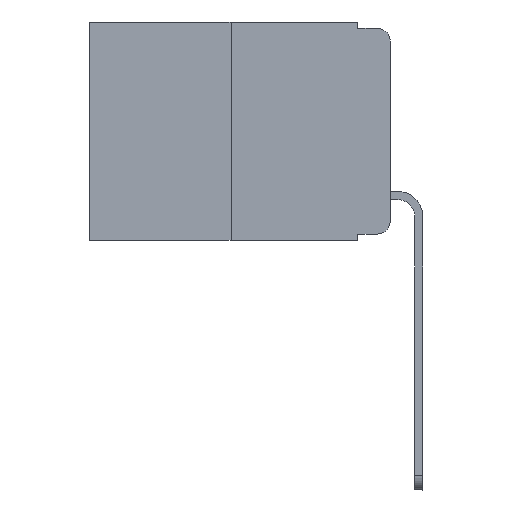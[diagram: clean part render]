
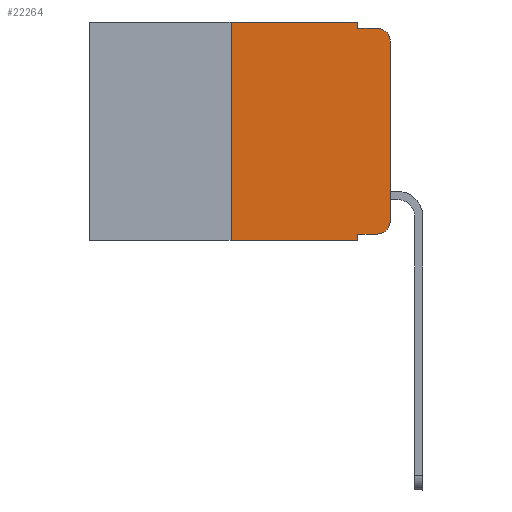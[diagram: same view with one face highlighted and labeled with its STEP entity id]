
A CAD part, left-side view. The second image highlights one B-rep face of the part: STEP entity #22264.
In plain terms, the highlighted planar face has unit normal (-1, 0, 0).
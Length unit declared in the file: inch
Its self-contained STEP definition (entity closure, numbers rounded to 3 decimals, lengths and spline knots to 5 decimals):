
#42 = EDGE_CURVE ( 'NONE', #20325, #2453, #16765, .T. ) ;
#64 = AXIS2_PLACEMENT_3D ( 'NONE', #23111, #12259, #12022 ) ;
#181 = FACE_OUTER_BOUND ( 'NONE', #1819, .T. ) ;
#229 = EDGE_CURVE ( 'NONE', #19959, #18418, #15147, .T. ) ;
#299 = DIRECTION ( 'NONE',  ( 0., -1., 0. ) ) ;
#469 = CARTESIAN_POINT ( 'NONE',  ( 0., 0.051, -0.343 ) ) ;
#717 = EDGE_CURVE ( 'NONE', #9767, #18418, #3385, .T. ) ;
#1424 = LINE ( 'NONE', #3088, #9580 ) ;
#1819 = EDGE_LOOP ( 'NONE', ( #15230, #8494, #3253, #11808, #14620, #3857, #10466, #4572, #10882, #14689 ) ) ;
#2147 = AXIS2_PLACEMENT_3D ( 'NONE', #18242, #2202, #5843 ) ;
#2202 = DIRECTION ( 'NONE',  ( 1., 0., 0. ) ) ;
#2453 = VERTEX_POINT ( 'NONE', #17876 ) ;
#3050 = EDGE_CURVE ( 'NONE', #20839, #9767, #3770, .T. ) ;
#3088 = CARTESIAN_POINT ( 'NONE',  ( 0., 0., 0. ) ) ;
#3138 = VERTEX_POINT ( 'NONE', #15104 ) ;
#3191 = VECTOR ( 'NONE', #299, 39.37008 ) ;
#3253 = ORIENTED_EDGE ( 'NONE', *, *, #717, .F. ) ;
#3354 = CARTESIAN_POINT ( 'NONE',  ( 0., 0.473, -0.343 ) ) ;
#3385 = LINE ( 'NONE', #10579, #3191 ) ;
#3426 = DIRECTION ( 'NONE',  ( 0., 0., -1. ) ) ;
#3770 = LINE ( 'NONE', #21583, #5003 ) ;
#3857 = ORIENTED_EDGE ( 'NONE', *, *, #22451, .F. ) ;
#4195 = LINE ( 'NONE', #20361, #11645 ) ;
#4379 = CARTESIAN_POINT ( 'NONE',  ( 0., 0.051, -0.333 ) ) ;
#4444 = LINE ( 'NONE', #17060, #19080 ) ;
#4572 = ORIENTED_EDGE ( 'NONE', *, *, #6352, .F. ) ;
#5003 = VECTOR ( 'NONE', #3426, 39.37008 ) ;
#5213 = CARTESIAN_POINT ( 'NONE',  ( 0., 0.02, -0.01 ) ) ;
#5234 = DIRECTION ( 'NONE',  ( 0., -1., 0. ) ) ;
#5843 = DIRECTION ( 'NONE',  ( 0., 0., -1. ) ) ;
#6077 = DIRECTION ( 'NONE',  ( 0., 0., 1. ) ) ;
#6222 = VERTEX_POINT ( 'NONE', #23311 ) ;
#6352 = EDGE_CURVE ( 'NONE', #20325, #15657, #4195, .T. ) ;
#6505 = DIRECTION ( 'NONE',  ( 0., 0., 1. ) ) ;
#6510 = CARTESIAN_POINT ( 'NONE',  ( 0., 0.25, 0. ) ) ;
#7336 = CIRCLE ( 'NONE', #11462, 0.02 ) ;
#8494 = ORIENTED_EDGE ( 'NONE', *, *, #229, .T. ) ;
#8700 = DIRECTION ( 'NONE',  ( -1., 0., 0. ) ) ;
#9149 = VERTEX_POINT ( 'NONE', #6510 ) ;
#9580 = VECTOR ( 'NONE', #6505, 39.37008 ) ;
#9767 = VERTEX_POINT ( 'NONE', #21343 ) ;
#10197 = DIRECTION ( 'NONE',  ( 0., -1., 0. ) ) ;
#10466 = ORIENTED_EDGE ( 'NONE', *, *, #17998, .T. ) ;
#10579 = CARTESIAN_POINT ( 'NONE',  ( 0., 0.051, -0.01 ) ) ;
#10882 = ORIENTED_EDGE ( 'NONE', *, *, #42, .T. ) ;
#11462 = AXIS2_PLACEMENT_3D ( 'NONE', #17684, #8700, #18522 ) ;
#11645 = VECTOR ( 'NONE', #21882, 39.37008 ) ;
#11808 = ORIENTED_EDGE ( 'NONE', *, *, #3050, .F. ) ;
#12022 = DIRECTION ( 'NONE',  ( 0., 0., -1. ) ) ;
#12259 = DIRECTION ( 'NONE',  ( -1., 0., 0. ) ) ;
#12309 = CARTESIAN_POINT ( 'NONE',  ( 0., 0.473, 0. ) ) ;
#12498 = CARTESIAN_POINT ( 'NONE',  ( 0., 0.051, -0.333 ) ) ;
#14196 = LINE ( 'NONE', #12309, #19074 ) ;
#14620 = ORIENTED_EDGE ( 'NONE', *, *, #15065, .F. ) ;
#14689 = ORIENTED_EDGE ( 'NONE', *, *, #18739, .T. ) ;
#15065 = EDGE_CURVE ( 'NONE', #9149, #20839, #14196, .T. ) ;
#15104 = CARTESIAN_POINT ( 'NONE',  ( 0., 0., -0.313 ) ) ;
#15147 = CIRCLE ( 'NONE', #64, 0.02 ) ;
#15230 = ORIENTED_EDGE ( 'NONE', *, *, #18453, .T. ) ;
#15657 = VERTEX_POINT ( 'NONE', #469 ) ;
#16343 = VECTOR ( 'NONE', #10197, 39.37008 ) ;
#16765 = LINE ( 'NONE', #4379, #22225 ) ;
#17060 = CARTESIAN_POINT ( 'NONE',  ( 0., 0.25, 0. ) ) ;
#17684 = CARTESIAN_POINT ( 'NONE',  ( 0., 0.02, -0.313 ) ) ;
#17839 = CARTESIAN_POINT ( 'NONE',  ( 0., 0., -0.03 ) ) ;
#17876 = CARTESIAN_POINT ( 'NONE',  ( 0., 0.02, -0.333 ) ) ;
#17998 = EDGE_CURVE ( 'NONE', #6222, #15657, #21156, .T. ) ;
#18242 = CARTESIAN_POINT ( 'NONE',  ( 0., 0.473, 0. ) ) ;
#18418 = VERTEX_POINT ( 'NONE', #5213 ) ;
#18453 = EDGE_CURVE ( 'NONE', #3138, #19959, #1424, .T. ) ;
#18522 = DIRECTION ( 'NONE',  ( 0., 0., -1. ) ) ;
#18739 = EDGE_CURVE ( 'NONE', #2453, #3138, #7336, .T. ) ;
#19074 = VECTOR ( 'NONE', #5234, 39.37008 ) ;
#19080 = VECTOR ( 'NONE', #6077, 39.37008 ) ;
#19429 = CARTESIAN_POINT ( 'NONE',  ( 0., 0.051, 0. ) ) ;
#19909 = PLANE ( 'NONE',  #2147 ) ;
#19959 = VERTEX_POINT ( 'NONE', #17839 ) ;
#20325 = VERTEX_POINT ( 'NONE', #12498 ) ;
#20361 = CARTESIAN_POINT ( 'NONE',  ( 0., 0.051, 0. ) ) ;
#20658 = DIRECTION ( 'NONE',  ( 0., -1., 0. ) ) ;
#20839 = VERTEX_POINT ( 'NONE', #19429 ) ;
#21156 = LINE ( 'NONE', #3354, #16343 ) ;
#21343 = CARTESIAN_POINT ( 'NONE',  ( 0., 0.051, -0.01 ) ) ;
#21583 = CARTESIAN_POINT ( 'NONE',  ( 0., 0.051, 0. ) ) ;
#21882 = DIRECTION ( 'NONE',  ( 0., 0., -1. ) ) ;
#22225 = VECTOR ( 'NONE', #20658, 39.37008 ) ;
#22264 = ADVANCED_FACE ( 'NONE', ( #181 ), #19909, .F. ) ;
#22451 = EDGE_CURVE ( 'NONE', #6222, #9149, #4444, .T. ) ;
#23111 = CARTESIAN_POINT ( 'NONE',  ( 0., 0.02, -0.03 ) ) ;
#23311 = CARTESIAN_POINT ( 'NONE',  ( 0., 0.25, -0.343 ) ) ;
